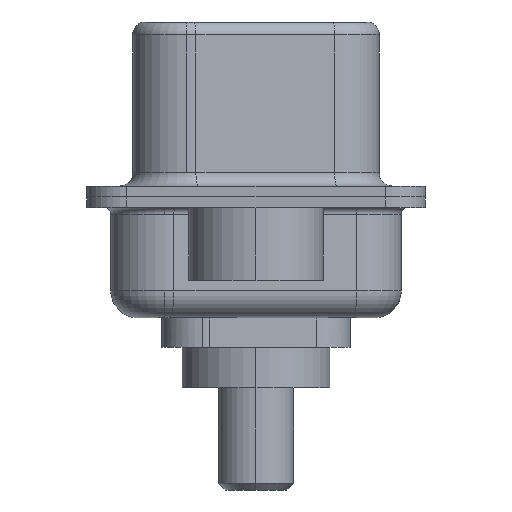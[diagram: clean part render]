
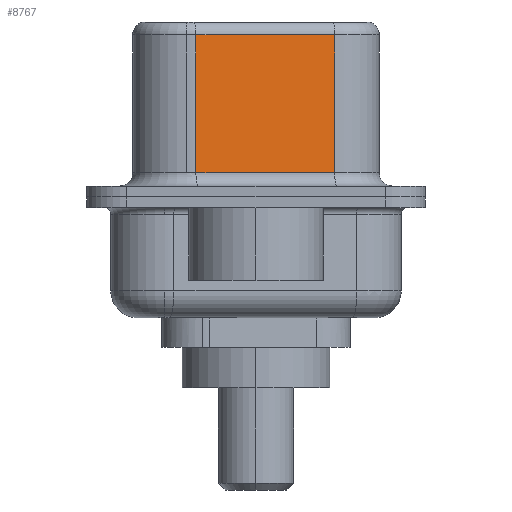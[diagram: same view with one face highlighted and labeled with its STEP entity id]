
A CAD part, left-side view. The second image highlights one B-rep face of the part: STEP entity #8767.
In plain terms, the highlighted planar face has unit normal (-0.985, -0.174, 0).
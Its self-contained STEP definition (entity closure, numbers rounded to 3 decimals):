
#248 = PLANE ( 'NONE',  #510 ) ;
#414 = LINE ( 'NONE', #7749, #18285 ) ;
#510 = AXIS2_PLACEMENT_3D ( 'NONE', #10268, #12505, #11615 ) ;
#1275 = LINE ( 'NONE', #13211, #12129 ) ;
#1992 = DIRECTION ( 'NONE',  ( 0., 0., -1. ) ) ;
#2047 = CARTESIAN_POINT ( 'NONE',  ( 3.655, 2.233, 0.9 ) ) ;
#2220 = FACE_OUTER_BOUND ( 'NONE', #3192, .T. ) ;
#3192 = EDGE_LOOP ( 'NONE', ( #13243, #17822, #9327, #5521 ) ) ;
#3700 = VERTEX_POINT ( 'NONE', #6831 ) ;
#3826 = LINE ( 'NONE', #18070, #18270 ) ;
#4608 = VERTEX_POINT ( 'NONE', #2047 ) ;
#4911 = DIRECTION ( 'NONE',  ( 0., 0., -1. ) ) ;
#5521 = ORIENTED_EDGE ( 'NONE', *, *, #14217, .T. ) ;
#6831 = CARTESIAN_POINT ( 'NONE',  ( 4.565, -2.927, 6.02 ) ) ;
#7362 = EDGE_CURVE ( 'NONE', #7795, #4608, #414, .T. ) ;
#7749 = CARTESIAN_POINT ( 'NONE',  ( 3.655, 2.233, 6.52 ) ) ;
#7795 = VERTEX_POINT ( 'NONE', #12698 ) ;
#8767 = ADVANCED_FACE ( 'NONE', ( #2220 ), #248, .F. ) ;
#9086 = DIRECTION ( 'NONE',  ( -0.174, 0.985, 0. ) ) ;
#9327 = ORIENTED_EDGE ( 'NONE', *, *, #7362, .T. ) ;
#9855 = EDGE_CURVE ( 'NONE', #3700, #16558, #1275, .T. ) ;
#10268 = CARTESIAN_POINT ( 'NONE',  ( 4.565, -2.927, 6.52 ) ) ;
#10623 = CARTESIAN_POINT ( 'NONE',  ( 4.565, -2.927, 0.9 ) ) ;
#11615 = DIRECTION ( 'NONE',  ( -0.174, 0.985, 0. ) ) ;
#12129 = VECTOR ( 'NONE', #4911, 1000. ) ;
#12505 = DIRECTION ( 'NONE',  ( 0.985, 0.174, 0. ) ) ;
#12698 = CARTESIAN_POINT ( 'NONE',  ( 3.655, 2.233, 6.02 ) ) ;
#13163 = CARTESIAN_POINT ( 'NONE',  ( 4.565, -2.927, 6.02 ) ) ;
#13211 = CARTESIAN_POINT ( 'NONE',  ( 4.565, -2.927, 6.52 ) ) ;
#13243 = ORIENTED_EDGE ( 'NONE', *, *, #9855, .F. ) ;
#13619 = VECTOR ( 'NONE', #9086, 1000. ) ;
#13910 = DIRECTION ( 'NONE',  ( 0.174, -0.985, 0. ) ) ;
#14217 = EDGE_CURVE ( 'NONE', #4608, #16558, #3826, .T. ) ;
#16558 = VERTEX_POINT ( 'NONE', #10623 ) ;
#17310 = LINE ( 'NONE', #13163, #13619 ) ;
#17790 = EDGE_CURVE ( 'NONE', #3700, #7795, #17310, .T. ) ;
#17822 = ORIENTED_EDGE ( 'NONE', *, *, #17790, .T. ) ;
#18070 = CARTESIAN_POINT ( 'NONE',  ( 4.565, -2.927, 0.9 ) ) ;
#18270 = VECTOR ( 'NONE', #13910, 1000. ) ;
#18285 = VECTOR ( 'NONE', #1992, 1000. ) ;
